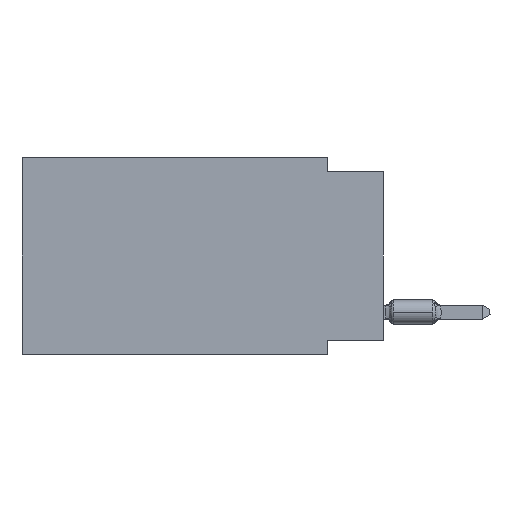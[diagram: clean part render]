
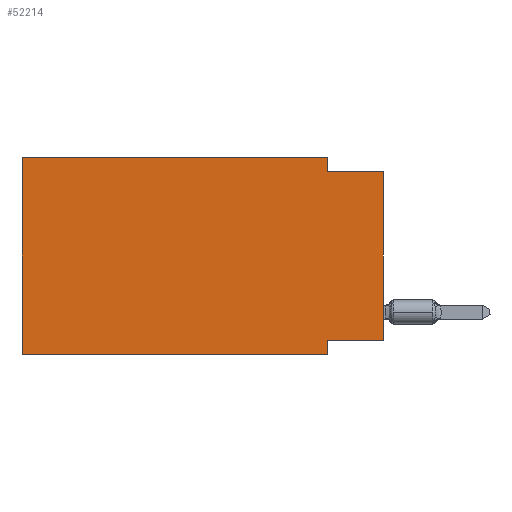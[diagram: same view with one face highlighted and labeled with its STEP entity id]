
A CAD part, left-side view. The second image highlights one B-rep face of the part: STEP entity #52214.
In plain terms, the highlighted planar face has unit normal (-1, 0, 0).
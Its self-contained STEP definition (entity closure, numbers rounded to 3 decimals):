
#634 = ORIENTED_EDGE ( 'NONE', *, *, #32982, .T. ) ;
#1810 = CARTESIAN_POINT ( 'NONE',  ( 0., 2.54, -8.255 ) ) ;
#2282 = CARTESIAN_POINT ( 'NONE',  ( 0., 16.383, 0. ) ) ;
#3424 = ORIENTED_EDGE ( 'NONE', *, *, #32482, .T. ) ;
#3794 = EDGE_CURVE ( 'NONE', #52518, #46263, #40105, .T. ) ;
#4036 = VERTEX_POINT ( 'NONE', #6218 ) ;
#5291 = LINE ( 'NONE', #55784, #34014 ) ;
#5933 = ORIENTED_EDGE ( 'NONE', *, *, #38967, .F. ) ;
#6218 = CARTESIAN_POINT ( 'NONE',  ( 0., 2.54, -8.89 ) ) ;
#9329 = LINE ( 'NONE', #35449, #35906 ) ;
#10450 = CARTESIAN_POINT ( 'NONE',  ( 0., 2.54, -0.635 ) ) ;
#12774 = VECTOR ( 'NONE', #46475, 1000. ) ;
#13692 = VERTEX_POINT ( 'NONE', #10450 ) ;
#15360 = EDGE_CURVE ( 'NONE', #17086, #4036, #44262, .T. ) ;
#15575 = DIRECTION ( 'NONE',  ( 0., -1., 0. ) ) ;
#16339 = VECTOR ( 'NONE', #17235, 1000. ) ;
#16539 = CARTESIAN_POINT ( 'NONE',  ( 0., 16.383, 0. ) ) ;
#17086 = VERTEX_POINT ( 'NONE', #1810 ) ;
#17235 = DIRECTION ( 'NONE',  ( 0., 0., 1. ) ) ;
#18053 = EDGE_CURVE ( 'NONE', #41457, #17086, #28320, .T. ) ;
#19095 = CARTESIAN_POINT ( 'NONE',  ( 0., 16.383, -8.89 ) ) ;
#19755 = EDGE_LOOP ( 'NONE', ( #3424, #5933, #21059, #29823, #30511, #634, #51653, #58612 ) ) ;
#20695 = FACE_OUTER_BOUND ( 'NONE', #19755, .T. ) ;
#21059 = ORIENTED_EDGE ( 'NONE', *, *, #27809, .F. ) ;
#21649 = DIRECTION ( 'NONE',  ( 0., 0., -1. ) ) ;
#24695 = AXIS2_PLACEMENT_3D ( 'NONE', #2282, #33759, #51914 ) ;
#25818 = CARTESIAN_POINT ( 'NONE',  ( 0., 2.54, -8.89 ) ) ;
#26165 = EDGE_CURVE ( 'NONE', #46263, #30928, #51290, .T. ) ;
#27186 = VECTOR ( 'NONE', #46540, 1000. ) ;
#27809 = EDGE_CURVE ( 'NONE', #30928, #13692, #5291, .T. ) ;
#28041 = LINE ( 'NONE', #38154, #28359 ) ;
#28320 = LINE ( 'NONE', #36947, #12774 ) ;
#28359 = VECTOR ( 'NONE', #15575, 1000. ) ;
#28586 = DIRECTION ( 'NONE',  ( 0., -1., 0. ) ) ;
#29731 = CARTESIAN_POINT ( 'NONE',  ( 0., 0., -0.635 ) ) ;
#29823 = ORIENTED_EDGE ( 'NONE', *, *, #26165, .F. ) ;
#30511 = ORIENTED_EDGE ( 'NONE', *, *, #3794, .F. ) ;
#30928 = VERTEX_POINT ( 'NONE', #36703 ) ;
#32482 = EDGE_CURVE ( 'NONE', #41457, #44426, #9329, .T. ) ;
#32982 = EDGE_CURVE ( 'NONE', #52518, #4036, #28041, .T. ) ;
#33192 = DIRECTION ( 'NONE',  ( 0., 0., -1. ) ) ;
#33759 = DIRECTION ( 'NONE',  ( 1., 0., 0. ) ) ;
#34014 = VECTOR ( 'NONE', #33192, 1000. ) ;
#35449 = CARTESIAN_POINT ( 'NONE',  ( 0., 0., 0. ) ) ;
#35906 = VECTOR ( 'NONE', #45577, 1000. ) ;
#36703 = CARTESIAN_POINT ( 'NONE',  ( 0., 2.54, 0. ) ) ;
#36947 = CARTESIAN_POINT ( 'NONE',  ( 0., 0., -8.255 ) ) ;
#37428 = CARTESIAN_POINT ( 'NONE',  ( 0., 0., -0.635 ) ) ;
#38154 = CARTESIAN_POINT ( 'NONE',  ( 0., 16.383, -8.89 ) ) ;
#38967 = EDGE_CURVE ( 'NONE', #13692, #44426, #42270, .T. ) ;
#39810 = CARTESIAN_POINT ( 'NONE',  ( 0., 16.383, 0. ) ) ;
#40105 = LINE ( 'NONE', #39810, #16339 ) ;
#41457 = VERTEX_POINT ( 'NONE', #57696 ) ;
#42270 = LINE ( 'NONE', #29731, #50199 ) ;
#44262 = LINE ( 'NONE', #25818, #52448 ) ;
#44426 = VERTEX_POINT ( 'NONE', #37428 ) ;
#45577 = DIRECTION ( 'NONE',  ( 0., 0., 1. ) ) ;
#45949 = CARTESIAN_POINT ( 'NONE',  ( 0., 16.383, 0. ) ) ;
#46263 = VERTEX_POINT ( 'NONE', #16539 ) ;
#46475 = DIRECTION ( 'NONE',  ( 0., 1., 0. ) ) ;
#46540 = DIRECTION ( 'NONE',  ( 0., -1., 0. ) ) ;
#50199 = VECTOR ( 'NONE', #28586, 1000. ) ;
#51290 = LINE ( 'NONE', #45949, #27186 ) ;
#51349 = PLANE ( 'NONE',  #24695 ) ;
#51653 = ORIENTED_EDGE ( 'NONE', *, *, #15360, .F. ) ;
#51914 = DIRECTION ( 'NONE',  ( 0., 0., -1. ) ) ;
#52214 = ADVANCED_FACE ( 'NONE', ( #20695 ), #51349, .F. ) ;
#52448 = VECTOR ( 'NONE', #21649, 1000. ) ;
#52518 = VERTEX_POINT ( 'NONE', #19095 ) ;
#55784 = CARTESIAN_POINT ( 'NONE',  ( 0., 2.54, 0. ) ) ;
#57696 = CARTESIAN_POINT ( 'NONE',  ( 0., 0., -8.255 ) ) ;
#58612 = ORIENTED_EDGE ( 'NONE', *, *, #18053, .F. ) ;
